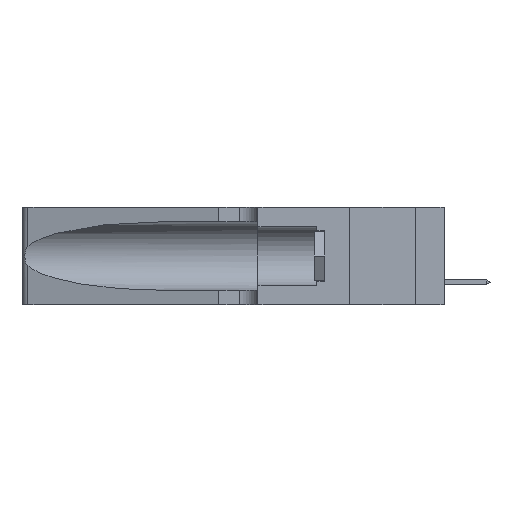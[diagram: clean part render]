
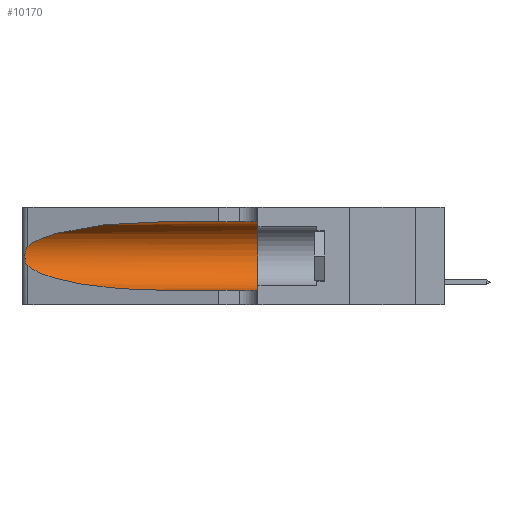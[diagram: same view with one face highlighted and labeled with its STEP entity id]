
A CAD part, left-side view. The second image highlights one B-rep face of the part: STEP entity #10170.
In plain terms, the highlighted cylindrical face has radius 3.308 mm (diameter 6.617 mm), a partial arc.
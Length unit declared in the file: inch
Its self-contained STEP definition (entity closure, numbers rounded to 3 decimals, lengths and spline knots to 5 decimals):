
#191 = CYLINDRICAL_SURFACE ( 'NONE', #22995, 0.13025 ) ;
#398 = VERTEX_POINT ( 'NONE', #14618 ) ;
#537 = DIRECTION ( 'NONE',  ( 0., 1., 0. ) ) ;
#1040 = VERTEX_POINT ( 'NONE', #3207 ) ;
#1375 = CARTESIAN_POINT ( 'NONE',  ( 0.25487, 1.22718, 0.14631 ) ) ;
#1416 = CARTESIAN_POINT ( 'NONE',  ( 0.26075, 1.23896, 0.178 ) ) ;
#1534 = CARTESIAN_POINT ( 'NONE',  ( 0.1305, 0.72297, 0.05475 ) ) ;
#2311 = CARTESIAN_POINT ( 'NONE',  ( 0.1305, 0.35, 0.185 ) ) ;
#2933 = B_SPLINE_CURVE_WITH_KNOTS ( 'NONE', 3,
 ( #23657, #8847, #9093, #14664, #20155, #18306, #10765, #1416, #18227, #21787, #7028, #22031, #20078, #10931 ),
 .UNSPECIFIED., .F., .F.,
 ( 4, 2, 2, 2, 2, 2, 4 ),
 ( 0., 0.00027, 0.00053, 0.00107, 0.0016, 0.00187, 0.00214 ),
 .UNSPECIFIED. ) ;
#2935 = CARTESIAN_POINT ( 'NONE',  ( 0.1305, 0.72297, 0.31525 ) ) ;
#3159 = CARTESIAN_POINT ( 'NONE',  ( 0.2373, 1.15595, 0.28018 ) ) ;
#3207 = CARTESIAN_POINT ( 'NONE',  ( 0.1305, 0.72297, 0.31525 ) ) ;
#3229 = CARTESIAN_POINT ( 'NONE',  ( 0.1305, 0.35, 0.05475 ) ) ;
#3303 = EDGE_CURVE ( 'NONE', #12381, #23242, #13925, .T. ) ;
#3743 = CARTESIAN_POINT ( 'NONE',  ( 0.25487, 1.22718, 0.14631 ) ) ;
#3782 = EDGE_CURVE ( 'NONE', #15953, #6283, #2933, .T. ) ;
#4243 = ORIENTED_EDGE ( 'NONE', *, *, #3782, .T. ) ;
#4899 = ORIENTED_EDGE ( 'NONE', *, *, #6834, .F. ) ;
#5097 = DIRECTION ( 'NONE',  ( 0., -1., 0. ) ) ;
#6059 = EDGE_CURVE ( 'NONE', #1040, #15953, #23111, .T. ) ;
#6063 = CARTESIAN_POINT ( 'NONE',  ( 0.1305, 0.72297, 0.05475 ) ) ;
#6283 = VERTEX_POINT ( 'NONE', #3743 ) ;
#6293 = FACE_OUTER_BOUND ( 'NONE', #7341, .T. ) ;
#6740 = CARTESIAN_POINT ( 'NONE',  ( 0.1305, 1.61858, 0.31525 ) ) ;
#6834 = EDGE_CURVE ( 'NONE', #1040, #398, #18949, .T. ) ;
#7028 = CARTESIAN_POINT ( 'NONE',  ( 0.25789, 1.23486, 0.15765 ) ) ;
#7206 = CARTESIAN_POINT ( 'NONE',  ( 0.1305, 1.61858, 0.185 ) ) ;
#7341 = EDGE_LOOP ( 'NONE', ( #14422, #4243, #11137, #7788, #13886, #4899 ) ) ;
#7788 = ORIENTED_EDGE ( 'NONE', *, *, #3303, .T. ) ;
#8847 = CARTESIAN_POINT ( 'NONE',  ( 0.25555, 1.22994, 0.2215 ) ) ;
#9093 = CARTESIAN_POINT ( 'NONE',  ( 0.25639, 1.23184, 0.21858 ) ) ;
#9140 = CIRCLE ( 'NONE', #20526, 0.13025 ) ;
#10170 = ADVANCED_FACE ( 'NONE', ( #6293 ), #191, .F. ) ;
#10714 = DIRECTION ( 'NONE',  ( 0., -1., 0. ) ) ;
#10765 = CARTESIAN_POINT ( 'NONE',  ( 0.26075, 1.23896, 0.19203 ) ) ;
#10864 = DIRECTION ( 'NONE',  ( 0., -1., 0. ) ) ;
#10931 = CARTESIAN_POINT ( 'NONE',  ( 0.25487, 1.22718, 0.14631 ) ) ;
#11137 = ORIENTED_EDGE ( 'NONE', *, *, #23312, .T. ) ;
#12227 = EDGE_CURVE ( 'NONE', #398, #23242, #9140, .T. ) ;
#12381 = VERTEX_POINT ( 'NONE', #6063 ) ;
#12455 = CARTESIAN_POINT ( 'NONE',  ( 0.25487, 1.22718, 0.22369 ) ) ;
#12585 = DIRECTION ( 'NONE',  ( 0., 0., -1. ) ) ;
#13249 = CARTESIAN_POINT ( 'NONE',  ( 0.1305, 1.61858, 0.05475 ) ) ;
#13629 = DIRECTION ( 'NONE',  ( 0., 0., 1. ) ) ;
#13886 = ORIENTED_EDGE ( 'NONE', *, *, #12227, .F. ) ;
#13925 = LINE ( 'NONE', #13249, #17692 ) ;
#14422 = ORIENTED_EDGE ( 'NONE', *, *, #6059, .T. ) ;
#14454 = CARTESIAN_POINT ( 'NONE',  ( 0.2373, 1.15595, 0.08982 ) ) ;
#14535 = CARTESIAN_POINT ( 'NONE',  ( 0.18966, 0.96281, 0.05475 ) ) ;
#14618 = CARTESIAN_POINT ( 'NONE',  ( 0.1305, 0.35, 0.31525 ) ) ;
#14664 = CARTESIAN_POINT ( 'NONE',  ( 0.25787, 1.23484, 0.2124 ) ) ;
#15953 = VERTEX_POINT ( 'NONE', #20419 ) ;
#16099 = CARTESIAN_POINT ( 'NONE',  ( 0.18966, 0.96281, 0.31525 ) ) ;
#16278 =( BOUNDED_CURVE ( )  B_SPLINE_CURVE ( 3, ( #1375, #14454, #14535, #1534 ),
 .UNSPECIFIED., .F., .F. ) 
 B_SPLINE_CURVE_WITH_KNOTS ( ( 4, 4 ),
 ( 3.44316, 4.71239 ),
 .UNSPECIFIED. ) 
 CURVE ( )  GEOMETRIC_REPRESENTATION_ITEM ( )  RATIONAL_B_SPLINE_CURVE ( ( 1., 0.87, 0.87, 1. ) ) 
 REPRESENTATION_ITEM ( '' )  );
#17692 = VECTOR ( 'NONE', #5097, 39.37008 ) ;
#18227 = CARTESIAN_POINT ( 'NONE',  ( 0.26017, 1.23833, 0.17102 ) ) ;
#18306 = CARTESIAN_POINT ( 'NONE',  ( 0.26018, 1.23835, 0.19895 ) ) ;
#18361 = VECTOR ( 'NONE', #10714, 39.37008 ) ;
#18949 = LINE ( 'NONE', #6740, #18361 ) ;
#20078 = CARTESIAN_POINT ( 'NONE',  ( 0.25555, 1.22993, 0.14849 ) ) ;
#20155 = CARTESIAN_POINT ( 'NONE',  ( 0.25854, 1.2359, 0.20912 ) ) ;
#20419 = CARTESIAN_POINT ( 'NONE',  ( 0.25487, 1.22718, 0.22369 ) ) ;
#20526 = AXIS2_PLACEMENT_3D ( 'NONE', #2311, #537, #13629 ) ;
#21787 = CARTESIAN_POINT ( 'NONE',  ( 0.25856, 1.23593, 0.16098 ) ) ;
#22031 = CARTESIAN_POINT ( 'NONE',  ( 0.25639, 1.23186, 0.15144 ) ) ;
#22995 = AXIS2_PLACEMENT_3D ( 'NONE', #7206, #10864, #12585 ) ;
#23111 =( BOUNDED_CURVE ( )  B_SPLINE_CURVE ( 3, ( #2935, #16099, #3159, #12455 ),
 .UNSPECIFIED., .F., .T. ) 
 B_SPLINE_CURVE_WITH_KNOTS ( ( 4, 4 ),
 ( 1.5708, 2.84003 ),
 .UNSPECIFIED. ) 
 CURVE ( )  GEOMETRIC_REPRESENTATION_ITEM ( )  RATIONAL_B_SPLINE_CURVE ( ( 1., 0.87, 0.87, 1. ) ) 
 REPRESENTATION_ITEM ( '' )  );
#23242 = VERTEX_POINT ( 'NONE', #3229 ) ;
#23312 = EDGE_CURVE ( 'NONE', #6283, #12381, #16278, .T. ) ;
#23657 = CARTESIAN_POINT ( 'NONE',  ( 0.25487, 1.22718, 0.22369 ) ) ;
